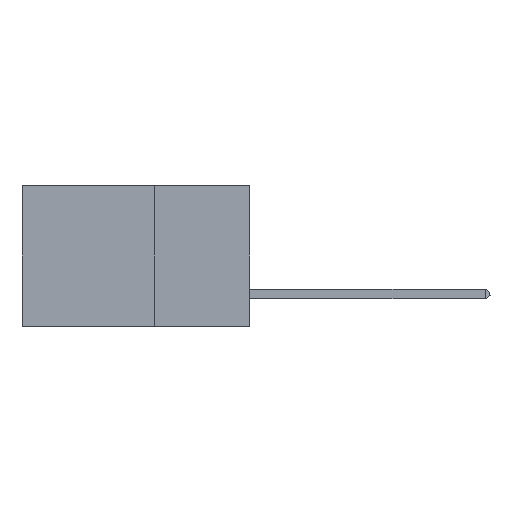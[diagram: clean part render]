
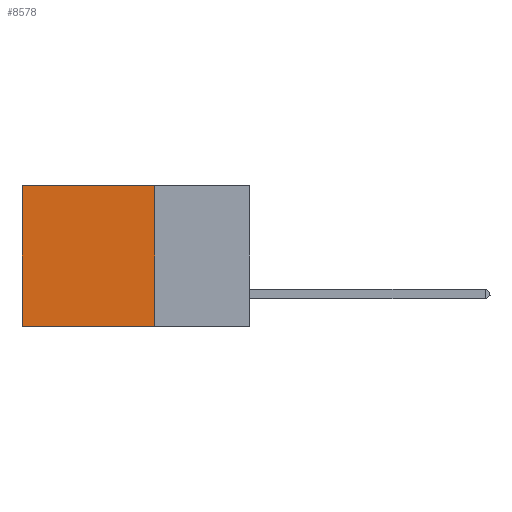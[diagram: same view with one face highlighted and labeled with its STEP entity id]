
A CAD part, left-side view. The second image highlights one B-rep face of the part: STEP entity #8578.
In plain terms, the highlighted planar face has unit normal (-1, 0, 0).
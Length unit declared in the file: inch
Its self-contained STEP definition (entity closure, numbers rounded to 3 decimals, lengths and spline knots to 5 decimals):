
#132 = EDGE_CURVE ( 'NONE', #14277, #14975, #11943, .T. ) ;
#139 = VERTEX_POINT ( 'NONE', #10362 ) ;
#774 = VECTOR ( 'NONE', #5357, 39.37008 ) ;
#924 = DIRECTION ( 'NONE',  ( 0., 0., -1. ) ) ;
#1698 = DIRECTION ( 'NONE',  ( 0., 0., -1. ) ) ;
#3185 = VECTOR ( 'NONE', #9948, 39.37008 ) ;
#3696 = CARTESIAN_POINT ( 'NONE',  ( 0.2875, 0.25, -0.37 ) ) ;
#3752 = LINE ( 'NONE', #11683, #774 ) ;
#4319 = ORIENTED_EDGE ( 'NONE', *, *, #132, .F. ) ;
#4985 = CARTESIAN_POINT ( 'NONE',  ( 0.2875, 0.25, 0. ) ) ;
#5357 = DIRECTION ( 'NONE',  ( 0., 1., 0. ) ) ;
#5675 = CARTESIAN_POINT ( 'NONE',  ( 0.2875, 0.25, 0. ) ) ;
#5711 = ORIENTED_EDGE ( 'NONE', *, *, #9086, .T. ) ;
#6706 = EDGE_CURVE ( 'NONE', #14975, #8430, #3752, .T. ) ;
#7123 = DIRECTION ( 'NONE',  ( 1., 0., 0. ) ) ;
#7413 = EDGE_LOOP ( 'NONE', ( #9953, #10752, #4319, #5711 ) ) ;
#7456 = CARTESIAN_POINT ( 'NONE',  ( 0.2875, 0.25, 0. ) ) ;
#7649 = LINE ( 'NONE', #7456, #3185 ) ;
#8311 = PLANE ( 'NONE',  #9462 ) ;
#8430 = VERTEX_POINT ( 'NONE', #9964 ) ;
#8578 = ADVANCED_FACE ( 'NONE', ( #10310 ), #8311, .F. ) ;
#8656 = CARTESIAN_POINT ( 'NONE',  ( 0.2875, 0.6, 0. ) ) ;
#9086 = EDGE_CURVE ( 'NONE', #14277, #139, #7649, .T. ) ;
#9462 = AXIS2_PLACEMENT_3D ( 'NONE', #12036, #7123, #924 ) ;
#9931 = EDGE_CURVE ( 'NONE', #139, #8430, #11025, .T. ) ;
#9948 = DIRECTION ( 'NONE',  ( 0., 1., 0. ) ) ;
#9953 = ORIENTED_EDGE ( 'NONE', *, *, #9931, .T. ) ;
#9964 = CARTESIAN_POINT ( 'NONE',  ( 0.2875, 0.6, -0.37 ) ) ;
#10001 = VECTOR ( 'NONE', #1698, 39.37008 ) ;
#10310 = FACE_OUTER_BOUND ( 'NONE', #7413, .T. ) ;
#10362 = CARTESIAN_POINT ( 'NONE',  ( 0.2875, 0.6, 0. ) ) ;
#10752 = ORIENTED_EDGE ( 'NONE', *, *, #6706, .F. ) ;
#11025 = LINE ( 'NONE', #8656, #12184 ) ;
#11683 = CARTESIAN_POINT ( 'NONE',  ( 0.2875, 0.25, -0.37 ) ) ;
#11943 = LINE ( 'NONE', #4985, #10001 ) ;
#12036 = CARTESIAN_POINT ( 'NONE',  ( 0.2875, 0.25, 0. ) ) ;
#12184 = VECTOR ( 'NONE', #12493, 39.37008 ) ;
#12493 = DIRECTION ( 'NONE',  ( 0., 0., -1. ) ) ;
#14277 = VERTEX_POINT ( 'NONE', #5675 ) ;
#14975 = VERTEX_POINT ( 'NONE', #3696 ) ;
